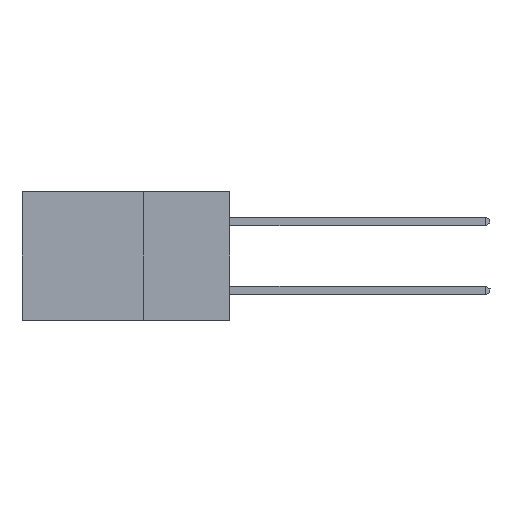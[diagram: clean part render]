
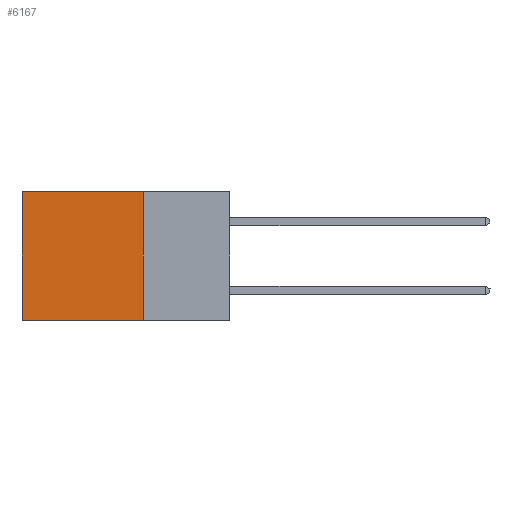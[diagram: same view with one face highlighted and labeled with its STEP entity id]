
A CAD part, left-side view. The second image highlights one B-rep face of the part: STEP entity #6167.
In plain terms, the highlighted planar face has unit normal (-1, 0, 0).
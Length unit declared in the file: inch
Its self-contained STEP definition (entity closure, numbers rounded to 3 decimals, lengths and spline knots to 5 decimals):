
#152 = VECTOR ( 'NONE', #1602, 39.37008 ) ;
#1272 = CARTESIAN_POINT ( 'NONE',  ( 0.298, 0.6, 0. ) ) ;
#1409 = AXIS2_PLACEMENT_3D ( 'NONE', #21046, #3761, #17267 ) ;
#1451 = PLANE ( 'NONE',  #1409 ) ;
#1602 = DIRECTION ( 'NONE',  ( 0., 0., -1. ) ) ;
#3434 = VERTEX_POINT ( 'NONE', #16141 ) ;
#3670 = LINE ( 'NONE', #1272, #21722 ) ;
#3761 = DIRECTION ( 'NONE',  ( 1., 0., 0. ) ) ;
#4696 = ORIENTED_EDGE ( 'NONE', *, *, #11787, .F. ) ;
#4719 = ORIENTED_EDGE ( 'NONE', *, *, #11675, .F. ) ;
#5598 = CARTESIAN_POINT ( 'NONE',  ( 0.298, 0.25, 0. ) ) ;
#6167 = ADVANCED_FACE ( 'NONE', ( #24250 ), #1451, .F. ) ;
#6995 = CARTESIAN_POINT ( 'NONE',  ( 0.298, 0.25, -0.37 ) ) ;
#7039 = DIRECTION ( 'NONE',  ( 0., 1., 0. ) ) ;
#7652 = VERTEX_POINT ( 'NONE', #10110 ) ;
#8663 = VECTOR ( 'NONE', #10290, 39.37008 ) ;
#8993 = DIRECTION ( 'NONE',  ( 0., 0., -1. ) ) ;
#9842 = LINE ( 'NONE', #16747, #25193 ) ;
#10110 = CARTESIAN_POINT ( 'NONE',  ( 0.298, 0.6, -0.37 ) ) ;
#10290 = DIRECTION ( 'NONE',  ( 0., 1., 0. ) ) ;
#11675 = EDGE_CURVE ( 'NONE', #17576, #20535, #15717, .T. ) ;
#11787 = EDGE_CURVE ( 'NONE', #20535, #7652, #16331, .T. ) ;
#12453 = ORIENTED_EDGE ( 'NONE', *, *, #16055, .T. ) ;
#15717 = LINE ( 'NONE', #5598, #152 ) ;
#16055 = EDGE_CURVE ( 'NONE', #3434, #7652, #3670, .T. ) ;
#16086 = EDGE_LOOP ( 'NONE', ( #12453, #4696, #4719, #23156 ) ) ;
#16141 = CARTESIAN_POINT ( 'NONE',  ( 0.298, 0.6, 0. ) ) ;
#16331 = LINE ( 'NONE', #17699, #8663 ) ;
#16577 = CARTESIAN_POINT ( 'NONE',  ( 0.298, 0.25, 0. ) ) ;
#16747 = CARTESIAN_POINT ( 'NONE',  ( 0.298, 0.25, 0. ) ) ;
#17267 = DIRECTION ( 'NONE',  ( 0., 0., -1. ) ) ;
#17576 = VERTEX_POINT ( 'NONE', #16577 ) ;
#17699 = CARTESIAN_POINT ( 'NONE',  ( 0.298, 0.25, -0.37 ) ) ;
#20535 = VERTEX_POINT ( 'NONE', #6995 ) ;
#21046 = CARTESIAN_POINT ( 'NONE',  ( 0.298, 0.25, 0. ) ) ;
#21722 = VECTOR ( 'NONE', #8993, 39.37008 ) ;
#23156 = ORIENTED_EDGE ( 'NONE', *, *, #24234, .T. ) ;
#24234 = EDGE_CURVE ( 'NONE', #17576, #3434, #9842, .T. ) ;
#24250 = FACE_OUTER_BOUND ( 'NONE', #16086, .T. ) ;
#25193 = VECTOR ( 'NONE', #7039, 39.37008 ) ;
